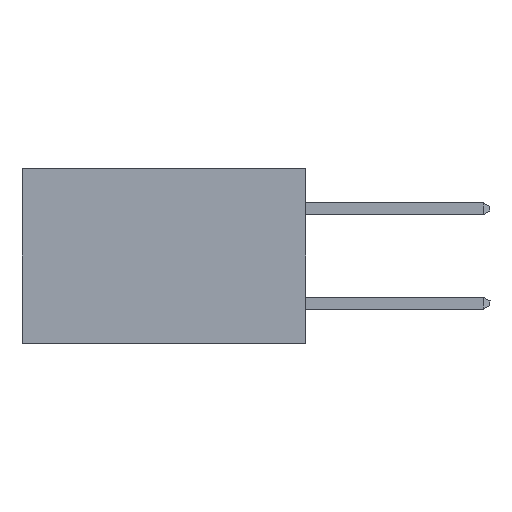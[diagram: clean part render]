
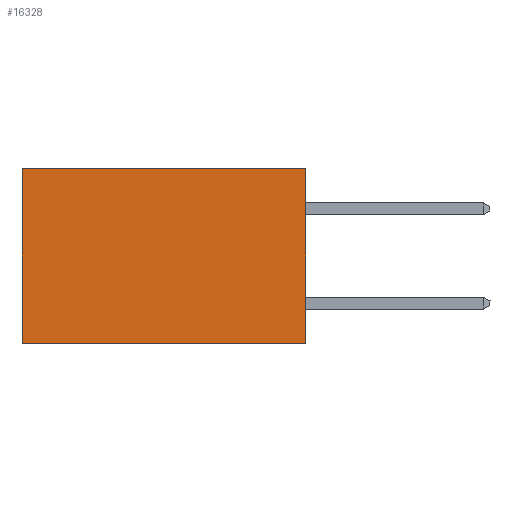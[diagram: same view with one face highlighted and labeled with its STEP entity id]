
A CAD part, left-side view. The second image highlights one B-rep face of the part: STEP entity #16328.
In plain terms, the highlighted planar face has unit normal (-1, 0, 0).
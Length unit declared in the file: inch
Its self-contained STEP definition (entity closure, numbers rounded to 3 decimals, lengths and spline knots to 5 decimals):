
#2496 = LINE ( 'NONE', #12500, #32298 ) ;
#3266 = EDGE_LOOP ( 'NONE', ( #5260, #27710, #9807, #24771 ) ) ;
#3374 = CARTESIAN_POINT ( 'NONE',  ( 0.298, 0., -0.37 ) ) ;
#4417 = EDGE_CURVE ( 'NONE', #17808, #25278, #13779, .T. ) ;
#4572 = PLANE ( 'NONE',  #21759 ) ;
#5260 = ORIENTED_EDGE ( 'NONE', *, *, #4417, .T. ) ;
#5707 = DIRECTION ( 'NONE',  ( 0., 1., 0. ) ) ;
#7027 = VECTOR ( 'NONE', #14847, 39.37008 ) ;
#7098 = CARTESIAN_POINT ( 'NONE',  ( 0.298, 0., 0. ) ) ;
#9807 = ORIENTED_EDGE ( 'NONE', *, *, #13105, .F. ) ;
#9944 = CARTESIAN_POINT ( 'NONE',  ( 0.298, 0.6, 0. ) ) ;
#12500 = CARTESIAN_POINT ( 'NONE',  ( 0.298, 0., 0. ) ) ;
#13105 = EDGE_CURVE ( 'NONE', #23279, #30307, #2496, .T. ) ;
#13779 = LINE ( 'NONE', #9944, #7027 ) ;
#13791 = CARTESIAN_POINT ( 'NONE',  ( 0.298, 0., 0. ) ) ;
#14007 = DIRECTION ( 'NONE',  ( 0., 1., 0. ) ) ;
#14063 = EDGE_CURVE ( 'NONE', #30307, #25278, #26909, .T. ) ;
#14847 = DIRECTION ( 'NONE',  ( 0., 0., -1. ) ) ;
#15001 = DIRECTION ( 'NONE',  ( 1., 0., 0. ) ) ;
#15984 = CARTESIAN_POINT ( 'NONE',  ( 0.298, 0., 0. ) ) ;
#16328 = ADVANCED_FACE ( 'NONE', ( #25167 ), #4572, .F. ) ;
#17350 = DIRECTION ( 'NONE',  ( 0., 0., -1. ) ) ;
#17808 = VERTEX_POINT ( 'NONE', #18074 ) ;
#18074 = CARTESIAN_POINT ( 'NONE',  ( 0.298, 0.6, 0. ) ) ;
#18258 = CARTESIAN_POINT ( 'NONE',  ( 0.298, 0.6, -0.37 ) ) ;
#18508 = VECTOR ( 'NONE', #14007, 39.37008 ) ;
#21759 = AXIS2_PLACEMENT_3D ( 'NONE', #7098, #15001, #17350 ) ;
#22881 = LINE ( 'NONE', #13791, #18508 ) ;
#23279 = VERTEX_POINT ( 'NONE', #15984 ) ;
#23749 = VECTOR ( 'NONE', #5707, 39.37008 ) ;
#24771 = ORIENTED_EDGE ( 'NONE', *, *, #30499, .T. ) ;
#25167 = FACE_OUTER_BOUND ( 'NONE', #3266, .T. ) ;
#25278 = VERTEX_POINT ( 'NONE', #18258 ) ;
#26909 = LINE ( 'NONE', #3374, #23749 ) ;
#27710 = ORIENTED_EDGE ( 'NONE', *, *, #14063, .F. ) ;
#30307 = VERTEX_POINT ( 'NONE', #32087 ) ;
#30472 = DIRECTION ( 'NONE',  ( 0., 0., -1. ) ) ;
#30499 = EDGE_CURVE ( 'NONE', #23279, #17808, #22881, .T. ) ;
#32087 = CARTESIAN_POINT ( 'NONE',  ( 0.298, 0., -0.37 ) ) ;
#32298 = VECTOR ( 'NONE', #30472, 39.37008 ) ;
